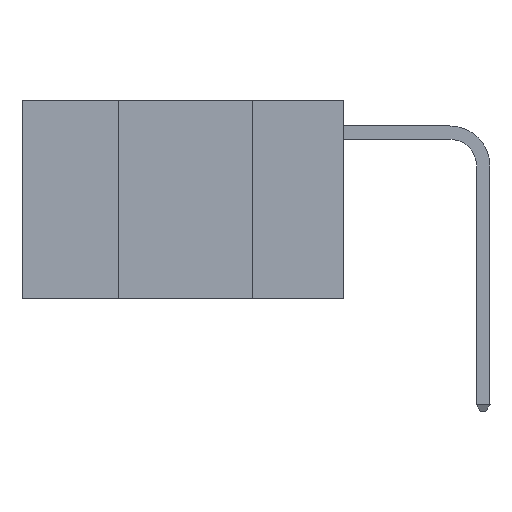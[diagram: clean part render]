
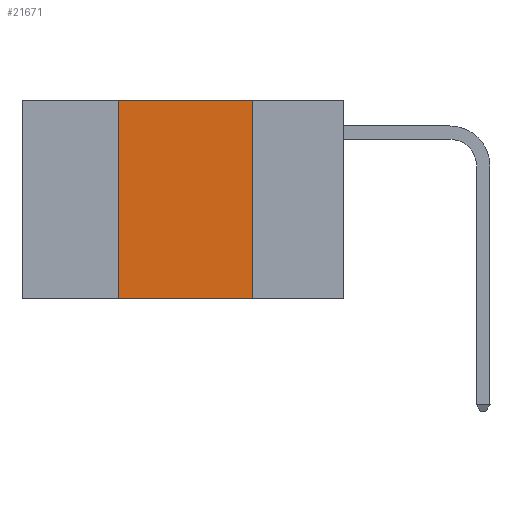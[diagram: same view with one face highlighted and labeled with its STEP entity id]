
A CAD part, left-side view. The second image highlights one B-rep face of the part: STEP entity #21671.
In plain terms, the highlighted planar face has unit normal (-1, 0, 0).
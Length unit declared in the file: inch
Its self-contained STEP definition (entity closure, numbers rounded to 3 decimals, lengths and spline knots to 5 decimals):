
#467 = CARTESIAN_POINT ( 'NONE',  ( 0., 0.6, -0.37 ) ) ;
#631 = DIRECTION ( 'NONE',  ( 0., 0., 1. ) ) ;
#1838 = PLANE ( 'NONE',  #21505 ) ;
#2316 = LINE ( 'NONE', #467, #22266 ) ;
#4018 = DIRECTION ( 'NONE',  ( 0., 0., -1. ) ) ;
#4520 = VERTEX_POINT ( 'NONE', #7051 ) ;
#4725 = VECTOR ( 'NONE', #22544, 39.37008 ) ;
#6322 = EDGE_CURVE ( 'NONE', #12288, #23418, #10081, .T. ) ;
#6787 = EDGE_LOOP ( 'NONE', ( #26522, #19636, #12832, #23044 ) ) ;
#7051 = CARTESIAN_POINT ( 'NONE',  ( 0., 0.42, 0. ) ) ;
#7369 = CARTESIAN_POINT ( 'NONE',  ( 0., 0.42, 0. ) ) ;
#8606 = VECTOR ( 'NONE', #631, 39.37008 ) ;
#10081 = LINE ( 'NONE', #16954, #22063 ) ;
#10930 = CARTESIAN_POINT ( 'NONE',  ( 0., 0.6, 0. ) ) ;
#11700 = DIRECTION ( 'NONE',  ( 0., -1., 0. ) ) ;
#12288 = VERTEX_POINT ( 'NONE', #15945 ) ;
#12296 = EDGE_CURVE ( 'NONE', #4520, #12288, #20531, .T. ) ;
#12531 = EDGE_CURVE ( 'NONE', #27768, #4520, #18863, .T. ) ;
#12832 = ORIENTED_EDGE ( 'NONE', *, *, #12531, .F. ) ;
#14240 = CARTESIAN_POINT ( 'NONE',  ( 0., 0.42, -0.37 ) ) ;
#15939 = CARTESIAN_POINT ( 'NONE',  ( 0., 0.6, 0. ) ) ;
#15945 = CARTESIAN_POINT ( 'NONE',  ( 0., 0.17, 0. ) ) ;
#16954 = CARTESIAN_POINT ( 'NONE',  ( 0., 0.17, 0. ) ) ;
#18863 = LINE ( 'NONE', #7369, #8606 ) ;
#19636 = ORIENTED_EDGE ( 'NONE', *, *, #12296, .F. ) ;
#20531 = LINE ( 'NONE', #10930, #4725 ) ;
#21505 = AXIS2_PLACEMENT_3D ( 'NONE', #15939, #25252, #4018 ) ;
#21671 = ADVANCED_FACE ( 'NONE', ( #22690 ), #1838, .F. ) ;
#22063 = VECTOR ( 'NONE', #28834, 39.37008 ) ;
#22266 = VECTOR ( 'NONE', #11700, 39.37008 ) ;
#22544 = DIRECTION ( 'NONE',  ( 0., -1., 0. ) ) ;
#22690 = FACE_OUTER_BOUND ( 'NONE', #6787, .T. ) ;
#23044 = ORIENTED_EDGE ( 'NONE', *, *, #29591, .T. ) ;
#23418 = VERTEX_POINT ( 'NONE', #25524 ) ;
#25252 = DIRECTION ( 'NONE',  ( 1., 0., 0. ) ) ;
#25524 = CARTESIAN_POINT ( 'NONE',  ( 0., 0.17, -0.37 ) ) ;
#26522 = ORIENTED_EDGE ( 'NONE', *, *, #6322, .F. ) ;
#27768 = VERTEX_POINT ( 'NONE', #14240 ) ;
#28834 = DIRECTION ( 'NONE',  ( 0., 0., -1. ) ) ;
#29591 = EDGE_CURVE ( 'NONE', #27768, #23418, #2316, .T. ) ;
